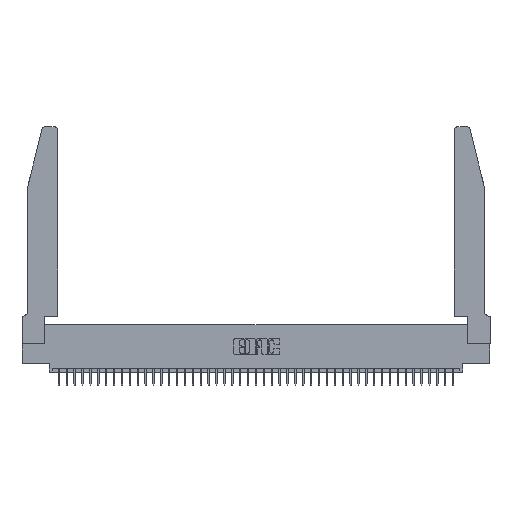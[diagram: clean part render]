
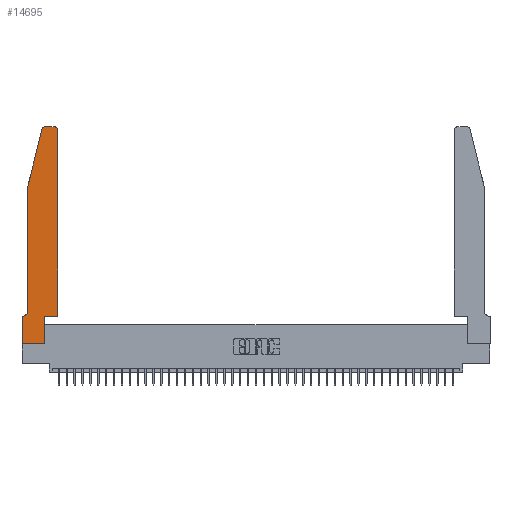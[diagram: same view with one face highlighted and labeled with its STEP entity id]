
A CAD part, top view. The second image highlights one B-rep face of the part: STEP entity #14695.
In plain terms, the highlighted planar face has unit normal (0, 0, 1).
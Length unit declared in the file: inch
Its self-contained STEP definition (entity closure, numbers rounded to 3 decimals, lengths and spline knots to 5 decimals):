
#111 = CARTESIAN_POINT ( 'NONE',  ( 0.25487, 2.72718, 0.37 ) ) ;
#894 = DIRECTION ( 'NONE',  ( 0., 0., -1. ) ) ;
#2389 = CARTESIAN_POINT ( 'NONE',  ( 0.0755, 2., 0.37 ) ) ;
#3007 = LINE ( 'NONE', #27146, #37974 ) ;
#4361 = DIRECTION ( 'NONE',  ( 1., 0., 0. ) ) ;
#4857 = AXIS2_PLACEMENT_3D ( 'NONE', #17262, #40720, #20636 ) ;
#4952 = DIRECTION ( 'NONE',  ( 0., 0., 1. ) ) ;
#5173 = CIRCLE ( 'NONE', #25992, 0.03 ) ;
#5797 = VECTOR ( 'NONE', #4361, 39.37008 ) ;
#5857 = DIRECTION ( 'NONE',  ( 0., -1., 0. ) ) ;
#6813 = DIRECTION ( 'NONE',  ( 0., -1., 0. ) ) ;
#6837 = CARTESIAN_POINT ( 'NONE',  ( 0.4505, 0.35, 0.37 ) ) ;
#7015 = CARTESIAN_POINT ( 'NONE',  ( 0.0755, 2., 0.37 ) ) ;
#7033 = EDGE_LOOP ( 'NONE', ( #35087, #22984, #19860, #24825, #37320, #10685, #9428, #32240, #36976, #32905, #33662, #37222 ) ) ;
#7127 = VERTEX_POINT ( 'NONE', #16516 ) ;
#7614 = VERTEX_POINT ( 'NONE', #12615 ) ;
#7906 = VERTEX_POINT ( 'NONE', #24281 ) ;
#8876 = DIRECTION ( 'NONE',  ( 0., 0., 1. ) ) ;
#9396 = EDGE_CURVE ( 'NONE', #7614, #24185, #26970, .T. ) ;
#9428 = ORIENTED_EDGE ( 'NONE', *, *, #31910, .T. ) ;
#10372 = LINE ( 'NONE', #7015, #36209 ) ;
#10685 = ORIENTED_EDGE ( 'NONE', *, *, #26326, .T. ) ;
#10842 = VECTOR ( 'NONE', #20492, 39.37008 ) ;
#11243 = VERTEX_POINT ( 'NONE', #43499 ) ;
#12615 = CARTESIAN_POINT ( 'NONE',  ( 0.2865, 0., 0.37 ) ) ;
#12991 = LINE ( 'NONE', #17110, #10842 ) ;
#13448 = EDGE_CURVE ( 'NONE', #30885, #7906, #26152, .T. ) ;
#13589 = DIRECTION ( 'NONE',  ( 0., 1., 0. ) ) ;
#14319 = DIRECTION ( 'NONE',  ( -1., 0., 0. ) ) ;
#14695 = ADVANCED_FACE ( 'NONE', ( #37017 ), #33982, .T. ) ;
#14837 = VECTOR ( 'NONE', #37263, 39.37008 ) ;
#14870 = EDGE_CURVE ( 'NONE', #29390, #7614, #22866, .T. ) ;
#15010 = AXIS2_PLACEMENT_3D ( 'NONE', #29141, #8876, #32499 ) ;
#15317 = EDGE_CURVE ( 'NONE', #32166, #7127, #31750, .T. ) ;
#15586 = EDGE_CURVE ( 'NONE', #7127, #11243, #5173, .T. ) ;
#16516 = CARTESIAN_POINT ( 'NONE',  ( 0.4505, 2.72, 0.37 ) ) ;
#16992 = CARTESIAN_POINT ( 'NONE',  ( 0.2865, 0.35, 0.37 ) ) ;
#17110 = CARTESIAN_POINT ( 'NONE',  ( 0.2605, 2.75, 0.37 ) ) ;
#17262 = CARTESIAN_POINT ( 'NONE',  ( 0., 0.35, 0.37 ) ) ;
#17456 = AXIS2_PLACEMENT_3D ( 'NONE', #21347, #894, #24731 ) ;
#17874 = LINE ( 'NONE', #41165, #43548 ) ;
#18286 = CARTESIAN_POINT ( 'NONE',  ( 0.4505, 0.35, 0.37 ) ) ;
#19860 = ORIENTED_EDGE ( 'NONE', *, *, #33981, .T. ) ;
#20492 = DIRECTION ( 'NONE',  ( -1., 0., 0. ) ) ;
#20636 = DIRECTION ( 'NONE',  ( 1., 0., 0. ) ) ;
#21347 = CARTESIAN_POINT ( 'NONE',  ( 0.0055, 0.42, 0.37 ) ) ;
#22821 = VECTOR ( 'NONE', #30243, 39.37008 ) ;
#22866 = LINE ( 'NONE', #34845, #5797 ) ;
#22984 = ORIENTED_EDGE ( 'NONE', *, *, #28653, .T. ) ;
#24185 = VERTEX_POINT ( 'NONE', #42067 ) ;
#24281 = CARTESIAN_POINT ( 'NONE',  ( 0.0055, 0.35, 0.37 ) ) ;
#24731 = DIRECTION ( 'NONE',  ( -1., 0., 0. ) ) ;
#24825 = ORIENTED_EDGE ( 'NONE', *, *, #40349, .T. ) ;
#24961 = CARTESIAN_POINT ( 'NONE',  ( 0.0755, 2., 0.37 ) ) ;
#25368 = CARTESIAN_POINT ( 'NONE',  ( 0.4205, 2.72, 0.37 ) ) ;
#25992 = AXIS2_PLACEMENT_3D ( 'NONE', #25368, #4952, #28752 ) ;
#26152 = CIRCLE ( 'NONE', #17456, 0.07 ) ;
#26326 = EDGE_CURVE ( 'NONE', #7906, #35820, #17874, .T. ) ;
#26806 = CARTESIAN_POINT ( 'NONE',  ( 0.0755, 0.42, 0.37 ) ) ;
#26970 = LINE ( 'NONE', #16992, #43664 ) ;
#27146 = CARTESIAN_POINT ( 'NONE',  ( 0., 0., 0.37 ) ) ;
#27439 = CARTESIAN_POINT ( 'NONE',  ( 0.284, 2.75, 0.37 ) ) ;
#28653 = EDGE_CURVE ( 'NONE', #32753, #41386, #35522, .T. ) ;
#28752 = DIRECTION ( 'NONE',  ( 1., 0., 0. ) ) ;
#29141 = CARTESIAN_POINT ( 'NONE',  ( 0.284, 2.72, 0.37 ) ) ;
#29390 = VERTEX_POINT ( 'NONE', #32581 ) ;
#30243 = DIRECTION ( 'NONE',  ( 0., 1., 0. ) ) ;
#30885 = VERTEX_POINT ( 'NONE', #26806 ) ;
#31750 = LINE ( 'NONE', #40166, #22821 ) ;
#31910 = EDGE_CURVE ( 'NONE', #35820, #29390, #3007, .T. ) ;
#32166 = VERTEX_POINT ( 'NONE', #18286 ) ;
#32240 = ORIENTED_EDGE ( 'NONE', *, *, #14870, .T. ) ;
#32379 = VECTOR ( 'NONE', #5857, 39.37008 ) ;
#32442 = VERTEX_POINT ( 'NONE', #24961 ) ;
#32499 = DIRECTION ( 'NONE',  ( 1., 0., 0. ) ) ;
#32581 = CARTESIAN_POINT ( 'NONE',  ( 0., 0., 0.37 ) ) ;
#32753 = VERTEX_POINT ( 'NONE', #27439 ) ;
#32905 = ORIENTED_EDGE ( 'NONE', *, *, #42006, .T. ) ;
#33662 = ORIENTED_EDGE ( 'NONE', *, *, #15317, .T. ) ;
#33762 = LINE ( 'NONE', #6837, #14837 ) ;
#33981 = EDGE_CURVE ( 'NONE', #41386, #32442, #10372, .T. ) ;
#33982 = PLANE ( 'NONE',  #4857 ) ;
#34034 = DIRECTION ( 'NONE',  ( -0.239, -0.971, 0. ) ) ;
#34629 = EDGE_CURVE ( 'NONE', #11243, #32753, #12991, .T. ) ;
#34845 = CARTESIAN_POINT ( 'NONE',  ( 0., 0., 0.37 ) ) ;
#35087 = ORIENTED_EDGE ( 'NONE', *, *, #34629, .T. ) ;
#35522 = CIRCLE ( 'NONE', #15010, 0.03 ) ;
#35820 = VERTEX_POINT ( 'NONE', #43292 ) ;
#36209 = VECTOR ( 'NONE', #34034, 39.37008 ) ;
#36976 = ORIENTED_EDGE ( 'NONE', *, *, #9396, .T. ) ;
#37017 = FACE_OUTER_BOUND ( 'NONE', #7033, .T. ) ;
#37222 = ORIENTED_EDGE ( 'NONE', *, *, #15586, .T. ) ;
#37263 = DIRECTION ( 'NONE',  ( 1., 0., 0. ) ) ;
#37320 = ORIENTED_EDGE ( 'NONE', *, *, #13448, .T. ) ;
#37974 = VECTOR ( 'NONE', #6813, 39.37008 ) ;
#40166 = CARTESIAN_POINT ( 'NONE',  ( 0.4505, 0.35, 0.37 ) ) ;
#40349 = EDGE_CURVE ( 'NONE', #32442, #30885, #42275, .T. ) ;
#40720 = DIRECTION ( 'NONE',  ( 0., 0., 1. ) ) ;
#41165 = CARTESIAN_POINT ( 'NONE',  ( 0.0755, 0.35, 0.37 ) ) ;
#41386 = VERTEX_POINT ( 'NONE', #111 ) ;
#42006 = EDGE_CURVE ( 'NONE', #24185, #32166, #33762, .T. ) ;
#42067 = CARTESIAN_POINT ( 'NONE',  ( 0.2865, 0.35, 0.37 ) ) ;
#42275 = LINE ( 'NONE', #2389, #32379 ) ;
#43292 = CARTESIAN_POINT ( 'NONE',  ( 0., 0.35, 0.37 ) ) ;
#43499 = CARTESIAN_POINT ( 'NONE',  ( 0.4205, 2.75, 0.37 ) ) ;
#43548 = VECTOR ( 'NONE', #14319, 39.37008 ) ;
#43664 = VECTOR ( 'NONE', #13589, 39.37008 ) ;
